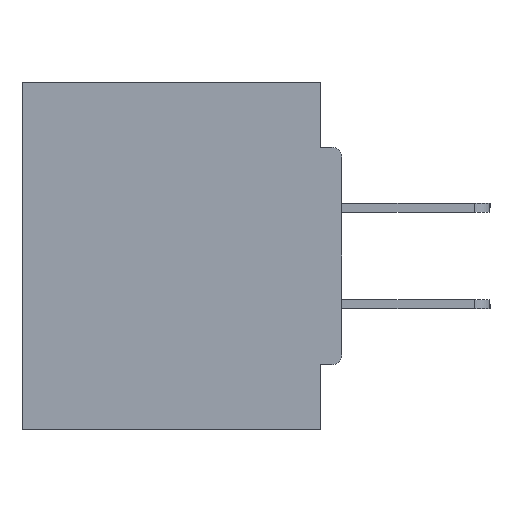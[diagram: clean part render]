
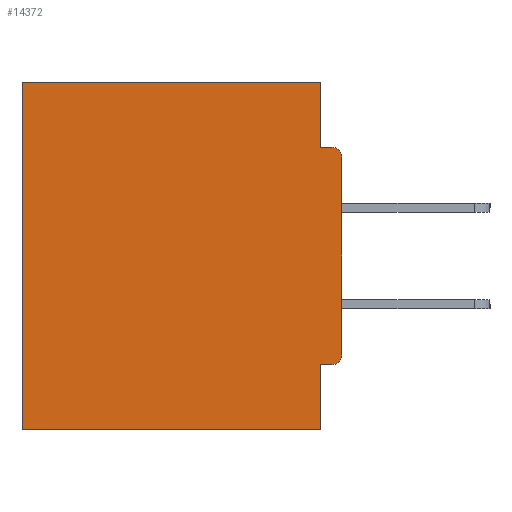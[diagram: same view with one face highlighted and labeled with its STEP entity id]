
A CAD part, left-side view. The second image highlights one B-rep face of the part: STEP entity #14372.
In plain terms, the highlighted planar face has unit normal (-1, 0, 0).
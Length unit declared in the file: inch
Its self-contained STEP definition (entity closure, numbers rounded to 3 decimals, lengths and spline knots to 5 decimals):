
#713 = VERTEX_POINT ( 'NONE', #29844 ) ;
#752 = DIRECTION ( 'NONE',  ( 0., 0., -1. ) ) ;
#871 = DIRECTION ( 'NONE',  ( -1., 0., 0. ) ) ;
#946 = CARTESIAN_POINT ( 'NONE',  ( 0.298, 0., 0. ) ) ;
#1280 = LINE ( 'NONE', #12857, #15058 ) ;
#1537 = EDGE_CURVE ( 'NONE', #29102, #3831, #31452, .T. ) ;
#1623 = CARTESIAN_POINT ( 'NONE',  ( 0.298, 0.015, -0.0935 ) ) ;
#1747 = DIRECTION ( 'NONE',  ( 0., 0., -1. ) ) ;
#1870 = DIRECTION ( 'NONE',  ( 1., 0., 0. ) ) ;
#2034 = EDGE_CURVE ( 'NONE', #29102, #29740, #23219, .T. ) ;
#2124 = ORIENTED_EDGE ( 'NONE', *, *, #17540, .F. ) ;
#2293 = CARTESIAN_POINT ( 'NONE',  ( 0.298, 0., 0. ) ) ;
#3831 = VERTEX_POINT ( 'NONE', #1623 ) ;
#4394 = AXIS2_PLACEMENT_3D ( 'NONE', #6575, #871, #752 ) ;
#4413 = VERTEX_POINT ( 'NONE', #5192 ) ;
#5192 = CARTESIAN_POINT ( 'NONE',  ( 0.298, 0.031, -0.5 ) ) ;
#5264 = CARTESIAN_POINT ( 'NONE',  ( 0.298, 0., -0.1085 ) ) ;
#6575 = CARTESIAN_POINT ( 'NONE',  ( 0.298, 0.015, -0.1085 ) ) ;
#6712 = EDGE_CURVE ( 'NONE', #16483, #25381, #30149, .T. ) ;
#7275 = LINE ( 'NONE', #25692, #28228 ) ;
#7558 = DIRECTION ( 'NONE',  ( 0., 0., -1. ) ) ;
#7571 = ORIENTED_EDGE ( 'NONE', *, *, #28758, .F. ) ;
#7718 = LINE ( 'NONE', #19180, #13299 ) ;
#7761 = ORIENTED_EDGE ( 'NONE', *, *, #6712, .T. ) ;
#8272 = DIRECTION ( 'NONE',  ( 0., -1., 0. ) ) ;
#9436 = LINE ( 'NONE', #24635, #30355 ) ;
#9575 = ORIENTED_EDGE ( 'NONE', *, *, #24382, .T. ) ;
#9585 = DIRECTION ( 'NONE',  ( 0., 0., -1. ) ) ;
#10302 = PLANE ( 'NONE',  #11351 ) ;
#11351 = AXIS2_PLACEMENT_3D ( 'NONE', #26449, #1870, #1747 ) ;
#12857 = CARTESIAN_POINT ( 'NONE',  ( 0.298, 0.031, -0.5 ) ) ;
#13069 = CARTESIAN_POINT ( 'NONE',  ( 0.298, 0.031, 0. ) ) ;
#13299 = VECTOR ( 'NONE', #16098, 39.37008 ) ;
#13738 = AXIS2_PLACEMENT_3D ( 'NONE', #28331, #23291, #22809 ) ;
#14372 = ADVANCED_FACE ( 'NONE', ( #15145 ), #10302, .F. ) ;
#14469 = VECTOR ( 'NONE', #26103, 39.37008 ) ;
#14657 = ORIENTED_EDGE ( 'NONE', *, *, #17916, .F. ) ;
#14773 = ORIENTED_EDGE ( 'NONE', *, *, #18771, .F. ) ;
#15058 = VECTOR ( 'NONE', #7558, 39.37008 ) ;
#15145 = FACE_OUTER_BOUND ( 'NONE', #29612, .T. ) ;
#15975 = VECTOR ( 'NONE', #21691, 39.37008 ) ;
#16098 = DIRECTION ( 'NONE',  ( 0., 0., -1. ) ) ;
#16483 = VERTEX_POINT ( 'NONE', #13069 ) ;
#16574 = EDGE_CURVE ( 'NONE', #32404, #3831, #9436, .T. ) ;
#16788 = EDGE_CURVE ( 'NONE', #22097, #29740, #24783, .T. ) ;
#17540 = EDGE_CURVE ( 'NONE', #19822, #4413, #7275, .T. ) ;
#17756 = DIRECTION ( 'NONE',  ( 0., 1., 0. ) ) ;
#17916 = EDGE_CURVE ( 'NONE', #4413, #713, #29835, .T. ) ;
#17975 = CARTESIAN_POINT ( 'NONE',  ( 0.298, 0.46, 0. ) ) ;
#18670 = CARTESIAN_POINT ( 'NONE',  ( 0.298, 0., -0.5 ) ) ;
#18771 = EDGE_CURVE ( 'NONE', #22097, #19822, #24258, .T. ) ;
#19180 = CARTESIAN_POINT ( 'NONE',  ( 0.298, 0.46, 0. ) ) ;
#19822 = VERTEX_POINT ( 'NONE', #28962 ) ;
#20656 = ORIENTED_EDGE ( 'NONE', *, *, #1537, .T. ) ;
#21691 = DIRECTION ( 'NONE',  ( 0., 0., -1. ) ) ;
#22097 = VERTEX_POINT ( 'NONE', #31071 ) ;
#22461 = VECTOR ( 'NONE', #17756, 39.37008 ) ;
#22698 = ORIENTED_EDGE ( 'NONE', *, *, #16788, .T. ) ;
#22809 = DIRECTION ( 'NONE',  ( 0., 0., -1. ) ) ;
#22847 = CARTESIAN_POINT ( 'NONE',  ( 0.298, 0., -0.4065 ) ) ;
#23219 = LINE ( 'NONE', #2293, #15975 ) ;
#23291 = DIRECTION ( 'NONE',  ( -1., 0., 0. ) ) ;
#23885 = VECTOR ( 'NONE', #29768, 39.37008 ) ;
#24258 = LINE ( 'NONE', #22847, #14469 ) ;
#24382 = EDGE_CURVE ( 'NONE', #25381, #713, #7718, .T. ) ;
#24598 = ORIENTED_EDGE ( 'NONE', *, *, #16574, .F. ) ;
#24635 = CARTESIAN_POINT ( 'NONE',  ( 0.298, 0., -0.0935 ) ) ;
#24783 = CIRCLE ( 'NONE', #13738, 0.015 ) ;
#25381 = VERTEX_POINT ( 'NONE', #17975 ) ;
#25692 = CARTESIAN_POINT ( 'NONE',  ( 0.298, 0.031, -0.5 ) ) ;
#26103 = DIRECTION ( 'NONE',  ( 0., 1., 0. ) ) ;
#26449 = CARTESIAN_POINT ( 'NONE',  ( 0.298, 0., 0. ) ) ;
#28228 = VECTOR ( 'NONE', #9585, 39.37008 ) ;
#28331 = CARTESIAN_POINT ( 'NONE',  ( 0.298, 0.015, -0.3915 ) ) ;
#28758 = EDGE_CURVE ( 'NONE', #16483, #32404, #1280, .T. ) ;
#28962 = CARTESIAN_POINT ( 'NONE',  ( 0.298, 0.031, -0.4065 ) ) ;
#29102 = VERTEX_POINT ( 'NONE', #5264 ) ;
#29150 = ORIENTED_EDGE ( 'NONE', *, *, #2034, .F. ) ;
#29612 = EDGE_LOOP ( 'NONE', ( #20656, #24598, #7571, #7761, #9575, #14657, #2124, #14773, #22698, #29150 ) ) ;
#29740 = VERTEX_POINT ( 'NONE', #32727 ) ;
#29768 = DIRECTION ( 'NONE',  ( 0., 1., 0. ) ) ;
#29835 = LINE ( 'NONE', #18670, #23885 ) ;
#29844 = CARTESIAN_POINT ( 'NONE',  ( 0.298, 0.46, -0.5 ) ) ;
#30149 = LINE ( 'NONE', #946, #22461 ) ;
#30355 = VECTOR ( 'NONE', #8272, 39.37008 ) ;
#31071 = CARTESIAN_POINT ( 'NONE',  ( 0.298, 0.015, -0.4065 ) ) ;
#31447 = CARTESIAN_POINT ( 'NONE',  ( 0.298, 0.031, -0.0935 ) ) ;
#31452 = CIRCLE ( 'NONE', #4394, 0.015 ) ;
#32404 = VERTEX_POINT ( 'NONE', #31447 ) ;
#32727 = CARTESIAN_POINT ( 'NONE',  ( 0.298, 0., -0.3915 ) ) ;
